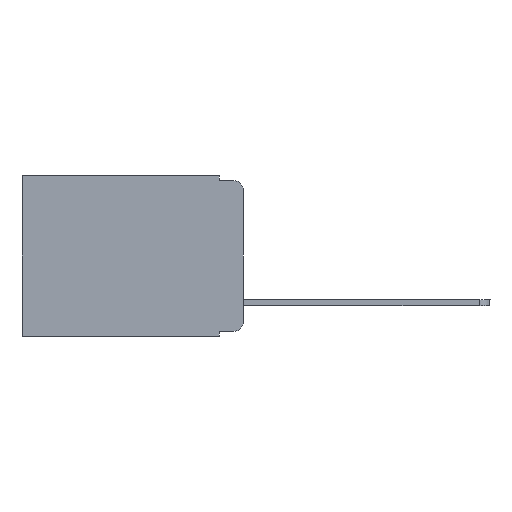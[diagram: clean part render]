
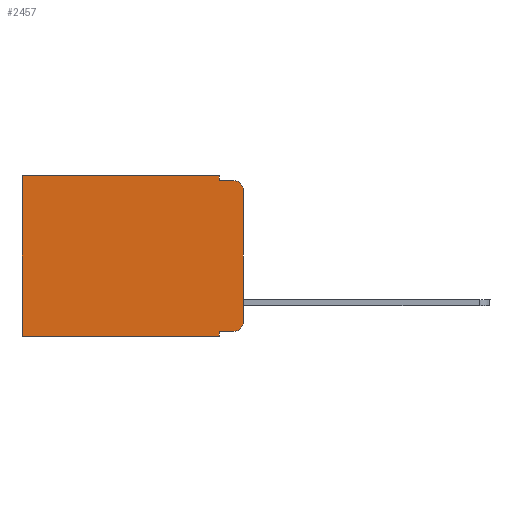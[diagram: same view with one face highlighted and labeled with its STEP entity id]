
A CAD part, left-side view. The second image highlights one B-rep face of the part: STEP entity #2457.
In plain terms, the highlighted planar face has unit normal (-1, 0, 0).
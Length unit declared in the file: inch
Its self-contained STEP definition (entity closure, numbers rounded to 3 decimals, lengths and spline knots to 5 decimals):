
#83 = CARTESIAN_POINT ( 'NONE',  ( 0.298, 0., -0.343 ) ) ;
#91 = VERTEX_POINT ( 'NONE', #11104 ) ;
#151 = DIRECTION ( 'NONE',  ( 0., -1., 0. ) ) ;
#297 = AXIS2_PLACEMENT_3D ( 'NONE', #6732, #1747, #8505 ) ;
#364 = EDGE_CURVE ( 'NONE', #4684, #9778, #1186, .T. ) ;
#534 = ORIENTED_EDGE ( 'NONE', *, *, #6499, .T. ) ;
#573 = EDGE_CURVE ( 'NONE', #9888, #10600, #6103, .T. ) ;
#687 = CARTESIAN_POINT ( 'NONE',  ( 0.298, 0.051, -0.01 ) ) ;
#926 = CARTESIAN_POINT ( 'NONE',  ( 0.298, 0.051, -0.343 ) ) ;
#936 = DIRECTION ( 'NONE',  ( 0., 0., -1. ) ) ;
#1143 = CARTESIAN_POINT ( 'NONE',  ( 0.298, 0.051, -0.01 ) ) ;
#1186 = CIRCLE ( 'NONE', #9569, 0.02 ) ;
#1459 = CARTESIAN_POINT ( 'NONE',  ( 0.298, 0., 0. ) ) ;
#1578 = DIRECTION ( 'NONE',  ( 0., 0., -1. ) ) ;
#1678 = ORIENTED_EDGE ( 'NONE', *, *, #8021, .F. ) ;
#1692 = EDGE_LOOP ( 'NONE', ( #11885, #4589, #1678, #9979, #534, #7175, #8844, #5964, #8108, #5692 ) ) ;
#1697 = VERTEX_POINT ( 'NONE', #687 ) ;
#1747 = DIRECTION ( 'NONE',  ( 1., 0., 0. ) ) ;
#2457 = ADVANCED_FACE ( 'NONE', ( #10588 ), #10659, .F. ) ;
#2629 = LINE ( 'NONE', #10749, #12286 ) ;
#2735 = CIRCLE ( 'NONE', #10263, 0.02 ) ;
#3179 = LINE ( 'NONE', #1143, #11008 ) ;
#3305 = DIRECTION ( 'NONE',  ( 0., 1., 0. ) ) ;
#3631 = DIRECTION ( 'NONE',  ( 0., 0., -1. ) ) ;
#3641 = EDGE_CURVE ( 'NONE', #7751, #10129, #2735, .T. ) ;
#4131 = DIRECTION ( 'NONE',  ( -1., 0., 0. ) ) ;
#4195 = VECTOR ( 'NONE', #6991, 39.37008 ) ;
#4474 = LINE ( 'NONE', #1459, #7272 ) ;
#4589 = ORIENTED_EDGE ( 'NONE', *, *, #364, .T. ) ;
#4684 = VERTEX_POINT ( 'NONE', #6029 ) ;
#4736 = VECTOR ( 'NONE', #7544, 39.37008 ) ;
#4988 = EDGE_CURVE ( 'NONE', #9888, #7751, #6544, .T. ) ;
#5314 = DIRECTION ( 'NONE',  ( 0., 0., -1. ) ) ;
#5692 = ORIENTED_EDGE ( 'NONE', *, *, #3641, .T. ) ;
#5934 = LINE ( 'NONE', #83, #8296 ) ;
#5964 = ORIENTED_EDGE ( 'NONE', *, *, #573, .F. ) ;
#5997 = CARTESIAN_POINT ( 'NONE',  ( 0.298, 0.051, 0. ) ) ;
#6029 = CARTESIAN_POINT ( 'NONE',  ( 0.298, 0., -0.03 ) ) ;
#6103 = LINE ( 'NONE', #6902, #8728 ) ;
#6499 = EDGE_CURVE ( 'NONE', #10293, #6824, #12737, .T. ) ;
#6544 = LINE ( 'NONE', #11387, #4736 ) ;
#6732 = CARTESIAN_POINT ( 'NONE',  ( 0.298, 0., 0. ) ) ;
#6786 = DIRECTION ( 'NONE',  ( 0., 1., 0. ) ) ;
#6824 = VERTEX_POINT ( 'NONE', #12455 ) ;
#6902 = CARTESIAN_POINT ( 'NONE',  ( 0.298, 0.051, 0. ) ) ;
#6990 = CARTESIAN_POINT ( 'NONE',  ( 0.298, 0.02, -0.333 ) ) ;
#6991 = DIRECTION ( 'NONE',  ( 0., 0., -1. ) ) ;
#7132 = CARTESIAN_POINT ( 'NONE',  ( 0.298, 0.051, -0.333 ) ) ;
#7175 = ORIENTED_EDGE ( 'NONE', *, *, #9154, .T. ) ;
#7272 = VECTOR ( 'NONE', #11465, 39.37008 ) ;
#7544 = DIRECTION ( 'NONE',  ( 0., -1., 0. ) ) ;
#7751 = VERTEX_POINT ( 'NONE', #6990 ) ;
#7906 = EDGE_CURVE ( 'NONE', #10600, #91, #5934, .T. ) ;
#7968 = LINE ( 'NONE', #5997, #4195 ) ;
#8021 = EDGE_CURVE ( 'NONE', #1697, #9778, #3179, .T. ) ;
#8108 = ORIENTED_EDGE ( 'NONE', *, *, #4988, .T. ) ;
#8153 = CARTESIAN_POINT ( 'NONE',  ( 0.298, 0.051, 0. ) ) ;
#8296 = VECTOR ( 'NONE', #3305, 39.37008 ) ;
#8505 = DIRECTION ( 'NONE',  ( 0., 0., -1. ) ) ;
#8531 = EDGE_CURVE ( 'NONE', #4684, #10129, #4474, .T. ) ;
#8728 = VECTOR ( 'NONE', #936, 39.37008 ) ;
#8844 = ORIENTED_EDGE ( 'NONE', *, *, #7906, .F. ) ;
#9154 = EDGE_CURVE ( 'NONE', #6824, #91, #2629, .T. ) ;
#9569 = AXIS2_PLACEMENT_3D ( 'NONE', #12588, #11792, #3631 ) ;
#9778 = VERTEX_POINT ( 'NONE', #11827 ) ;
#9867 = CARTESIAN_POINT ( 'NONE',  ( 0.298, 0., 0. ) ) ;
#9888 = VERTEX_POINT ( 'NONE', #7132 ) ;
#9979 = ORIENTED_EDGE ( 'NONE', *, *, #11389, .F. ) ;
#10129 = VERTEX_POINT ( 'NONE', #10848 ) ;
#10263 = AXIS2_PLACEMENT_3D ( 'NONE', #12168, #4131, #5314 ) ;
#10293 = VERTEX_POINT ( 'NONE', #8153 ) ;
#10588 = FACE_OUTER_BOUND ( 'NONE', #1692, .T. ) ;
#10600 = VERTEX_POINT ( 'NONE', #926 ) ;
#10659 = PLANE ( 'NONE',  #297 ) ;
#10749 = CARTESIAN_POINT ( 'NONE',  ( 0.298, 0.473, 0. ) ) ;
#10848 = CARTESIAN_POINT ( 'NONE',  ( 0.298, 0., -0.313 ) ) ;
#11008 = VECTOR ( 'NONE', #151, 39.37008 ) ;
#11104 = CARTESIAN_POINT ( 'NONE',  ( 0.298, 0.473, -0.343 ) ) ;
#11387 = CARTESIAN_POINT ( 'NONE',  ( 0.298, 0.051, -0.333 ) ) ;
#11389 = EDGE_CURVE ( 'NONE', #10293, #1697, #7968, .T. ) ;
#11465 = DIRECTION ( 'NONE',  ( 0., 0., -1. ) ) ;
#11792 = DIRECTION ( 'NONE',  ( -1., 0., 0. ) ) ;
#11827 = CARTESIAN_POINT ( 'NONE',  ( 0.298, 0.02, -0.01 ) ) ;
#11885 = ORIENTED_EDGE ( 'NONE', *, *, #8531, .F. ) ;
#12168 = CARTESIAN_POINT ( 'NONE',  ( 0.298, 0.02, -0.313 ) ) ;
#12286 = VECTOR ( 'NONE', #1578, 39.37008 ) ;
#12355 = VECTOR ( 'NONE', #6786, 39.37008 ) ;
#12455 = CARTESIAN_POINT ( 'NONE',  ( 0.298, 0.473, 0. ) ) ;
#12588 = CARTESIAN_POINT ( 'NONE',  ( 0.298, 0.02, -0.03 ) ) ;
#12737 = LINE ( 'NONE', #9867, #12355 ) ;
